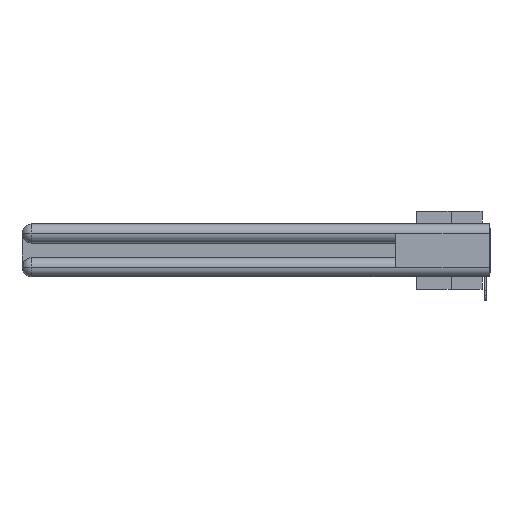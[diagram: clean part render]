
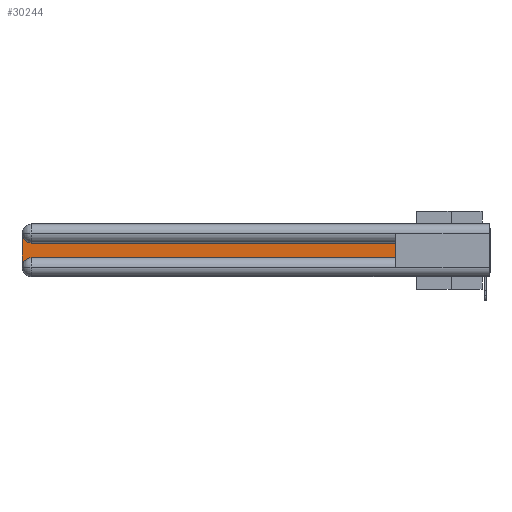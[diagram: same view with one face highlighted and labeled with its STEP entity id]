
A CAD part, left-side view. The second image highlights one B-rep face of the part: STEP entity #30244.
In plain terms, the highlighted planar face has unit normal (-1, 0, 0).
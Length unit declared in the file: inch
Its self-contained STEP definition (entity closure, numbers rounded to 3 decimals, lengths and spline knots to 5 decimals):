
#695 = CARTESIAN_POINT ( 'NONE',  ( 0.075, 3., -0.0625 ) ) ;
#2017 = CIRCLE ( 'NONE', #19627, 0.06 ) ;
#2636 = AXIS2_PLACEMENT_3D ( 'NONE', #27185, #19665, #27498 ) ;
#2688 = CARTESIAN_POINT ( 'NONE',  ( 0.075, 0.6, -0.2175 ) ) ;
#4007 = DIRECTION ( 'NONE',  ( 0., 0., 1. ) ) ;
#4638 = ORIENTED_EDGE ( 'NONE', *, *, #19182, .T. ) ;
#5256 = VERTEX_POINT ( 'NONE', #2688 ) ;
#5467 = EDGE_CURVE ( 'NONE', #5256, #29681, #7011, .T. ) ;
#5603 = VERTEX_POINT ( 'NONE', #28053 ) ;
#5612 = LINE ( 'NONE', #28845, #11764 ) ;
#7011 = LINE ( 'NONE', #19712, #25289 ) ;
#7270 = ORIENTED_EDGE ( 'NONE', *, *, #15064, .T. ) ;
#7765 = VERTEX_POINT ( 'NONE', #31319 ) ;
#8340 = DIRECTION ( 'NONE',  ( 0., 0., -1. ) ) ;
#8852 = DIRECTION ( 'NONE',  ( 0., 0., -1. ) ) ;
#9987 = AXIS2_PLACEMENT_3D ( 'NONE', #23875, #24034, #8340 ) ;
#11764 = VECTOR ( 'NONE', #31165, 39.37008 ) ;
#12958 = DIRECTION ( 'NONE',  ( 1., 0., 0. ) ) ;
#14191 = VERTEX_POINT ( 'NONE', #695 ) ;
#15064 = EDGE_CURVE ( 'NONE', #5603, #5256, #31323, .T. ) ;
#15811 = ORIENTED_EDGE ( 'NONE', *, *, #5467, .T. ) ;
#16106 = DIRECTION ( 'NONE',  ( 0., -1., 0. ) ) ;
#16248 = ORIENTED_EDGE ( 'NONE', *, *, #18898, .T. ) ;
#16527 = CIRCLE ( 'NONE', #2636, 0.06 ) ;
#17307 = EDGE_CURVE ( 'NONE', #14191, #20248, #24209, .T. ) ;
#17790 = CARTESIAN_POINT ( 'NONE',  ( 0.075, 2.94, -0.0625 ) ) ;
#17923 = CARTESIAN_POINT ( 'NONE',  ( 0.075, 0.6, -0.1225 ) ) ;
#17950 = DIRECTION ( 'NONE',  ( 0., 0., -1. ) ) ;
#18889 = CARTESIAN_POINT ( 'NONE',  ( 0.075, 3., -0.2175 ) ) ;
#18898 = EDGE_CURVE ( 'NONE', #20248, #5603, #16527, .T. ) ;
#19182 = EDGE_CURVE ( 'NONE', #29681, #7765, #5612, .T. ) ;
#19627 = AXIS2_PLACEMENT_3D ( 'NONE', #17790, #12958, #17950 ) ;
#19665 = DIRECTION ( 'NONE',  ( 1., 0., 0. ) ) ;
#19712 = CARTESIAN_POINT ( 'NONE',  ( 0.075, 0.6, -0.2175 ) ) ;
#20248 = VERTEX_POINT ( 'NONE', #20323 ) ;
#20323 = CARTESIAN_POINT ( 'NONE',  ( 0.075, 3., -0.2775 ) ) ;
#21679 = EDGE_LOOP ( 'NONE', ( #4638, #32957, #27140, #16248, #7270, #15811 ) ) ;
#23875 = CARTESIAN_POINT ( 'NONE',  ( 0.075, 3., -0.1225 ) ) ;
#24034 = DIRECTION ( 'NONE',  ( 1., 0., 0. ) ) ;
#24192 = FACE_OUTER_BOUND ( 'NONE', #21679, .T. ) ;
#24209 = LINE ( 'NONE', #18889, #25499 ) ;
#25289 = VECTOR ( 'NONE', #4007, 39.37008 ) ;
#25499 = VECTOR ( 'NONE', #8852, 39.37008 ) ;
#25797 = CARTESIAN_POINT ( 'NONE',  ( 0.075, 0.6, -0.2175 ) ) ;
#27140 = ORIENTED_EDGE ( 'NONE', *, *, #17307, .T. ) ;
#27185 = CARTESIAN_POINT ( 'NONE',  ( 0.075, 2.94, -0.2775 ) ) ;
#27498 = DIRECTION ( 'NONE',  ( 0., 0., -1. ) ) ;
#28053 = CARTESIAN_POINT ( 'NONE',  ( 0.075, 2.94, -0.2175 ) ) ;
#28676 = VECTOR ( 'NONE', #16106, 39.37008 ) ;
#28845 = CARTESIAN_POINT ( 'NONE',  ( 0.075, 0.6, -0.1225 ) ) ;
#29681 = VERTEX_POINT ( 'NONE', #17923 ) ;
#30244 = ADVANCED_FACE ( 'NONE', ( #24192 ), #31222, .F. ) ;
#31112 = EDGE_CURVE ( 'NONE', #7765, #14191, #2017, .T. ) ;
#31165 = DIRECTION ( 'NONE',  ( 0., 1., 0. ) ) ;
#31222 = PLANE ( 'NONE',  #9987 ) ;
#31319 = CARTESIAN_POINT ( 'NONE',  ( 0.075, 2.94, -0.1225 ) ) ;
#31323 = LINE ( 'NONE', #25797, #28676 ) ;
#32957 = ORIENTED_EDGE ( 'NONE', *, *, #31112, .T. ) ;
